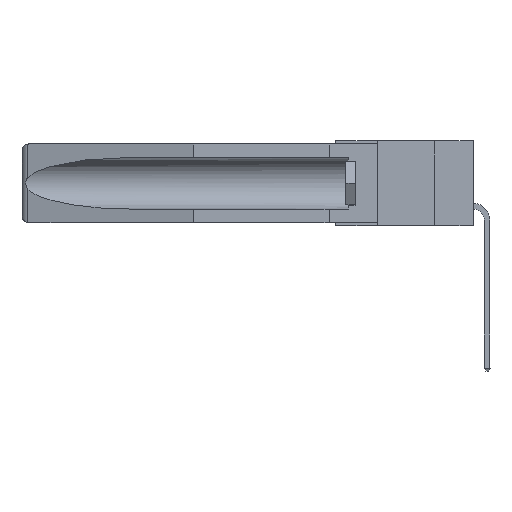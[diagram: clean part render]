
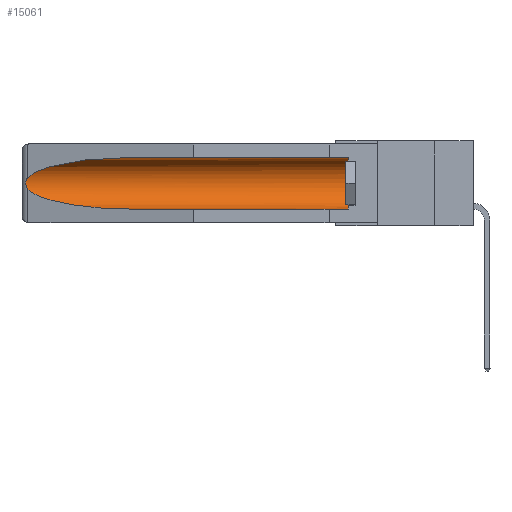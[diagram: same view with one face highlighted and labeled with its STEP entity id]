
A CAD part, left-side view. The second image highlights one B-rep face of the part: STEP entity #15061.
In plain terms, the highlighted cylindrical face has radius 2.857 mm (diameter 5.715 mm), a partial arc.
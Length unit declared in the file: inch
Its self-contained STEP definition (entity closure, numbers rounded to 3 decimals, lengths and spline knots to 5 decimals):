
#56 = VERTEX_POINT ( 'NONE', #14654 ) ;
#414 = AXIS2_PLACEMENT_3D ( 'NONE', #13241, #4403, #14778 ) ;
#901 = CARTESIAN_POINT ( 'NONE',  ( 0.21114, 1.30732, -0.284 ) ) ;
#962 = CARTESIAN_POINT ( 'NONE',  ( 0.25451, 1.48313, -0.09465 ) ) ;
#967 = CARTESIAN_POINT ( 'NONE',  ( 0.155, 1.07973, -0.284 ) ) ;
#1144 = DIRECTION ( 'NONE',  ( 0., 0., 1. ) ) ;
#1234 = FACE_OUTER_BOUND ( 'NONE', #15044, .T. ) ;
#1832 = LINE ( 'NONE', #9757, #6732 ) ;
#2042 = CARTESIAN_POINT ( 'NONE',  ( 0.26537, 1.52718, -0.19328 ) ) ;
#2167 = CARTESIAN_POINT ( 'NONE',  ( 0.26597, 1.52961, -0.15275 ) ) ;
#2314 = CARTESIAN_POINT ( 'NONE',  ( 0.26655, 1.53094, -0.18657 ) ) ;
#3698 = CARTESIAN_POINT ( 'NONE',  ( 0.2673, 1.53269, -0.17917 ) ) ;
#3832 = DIRECTION ( 'NONE',  ( 0., 1., 0. ) ) ;
#3889 = CIRCLE ( 'NONE', #11942, 0.1125 ) ;
#4142 = CARTESIAN_POINT ( 'NONE',  ( 0.26537, 1.52718, -0.14972 ) ) ;
#4305 = VERTEX_POINT ( 'NONE', #18230 ) ;
#4403 = DIRECTION ( 'NONE',  ( 0., 1., 0. ) ) ;
#4667 = LINE ( 'NONE', #8243, #4895 ) ;
#4740 = VERTEX_POINT ( 'NONE', #14899 ) ;
#4895 = VECTOR ( 'NONE', #8170, 39.37008 ) ;
#5308 = CARTESIAN_POINT ( 'NONE',  ( 0.26597, 1.5296, -0.19026 ) ) ;
#6732 = VECTOR ( 'NONE', #3832, 39.37008 ) ;
#6853 =( BOUNDED_CURVE ( )  B_SPLINE_CURVE ( 3, ( #8586, #9779, #901, #967 ),
 .UNSPECIFIED., .F., .T. ) 
 B_SPLINE_CURVE_WITH_KNOTS ( ( 4, 4 ),
 ( 0.1948, 1.5708 ),
 .UNSPECIFIED. ) 
 CURVE ( )  GEOMETRIC_REPRESENTATION_ITEM ( )  RATIONAL_B_SPLINE_CURVE ( ( 1., 0.848, 0.848, 1. ) ) 
 REPRESENTATION_ITEM ( '' )  );
#7014 = ORIENTED_EDGE ( 'NONE', *, *, #17585, .F. ) ;
#8170 = DIRECTION ( 'NONE',  ( 0., 1., 0. ) ) ;
#8243 = CARTESIAN_POINT ( 'NONE',  ( 0.155, -0.30754, -0.059 ) ) ;
#8586 = CARTESIAN_POINT ( 'NONE',  ( 0.26537, 1.52718, -0.19328 ) ) ;
#8675 = ORIENTED_EDGE ( 'NONE', *, *, #17444, .T. ) ;
#9653 = CARTESIAN_POINT ( 'NONE',  ( 0.2675, 1.53308, -0.17534 ) ) ;
#9757 = CARTESIAN_POINT ( 'NONE',  ( 0.155, -0.30754, -0.284 ) ) ;
#9779 = CARTESIAN_POINT ( 'NONE',  ( 0.25451, 1.48313, -0.24835 ) ) ;
#10020 = CARTESIAN_POINT ( 'NONE',  ( 0.155, 0.126, -0.1715 ) ) ;
#10242 =( BOUNDED_CURVE ( )  B_SPLINE_CURVE ( 3, ( #18774, #12919, #962, #4142 ),
 .UNSPECIFIED., .F., .F. ) 
 B_SPLINE_CURVE_WITH_KNOTS ( ( 4, 4 ),
 ( 4.71239, 6.08839 ),
 .UNSPECIFIED. ) 
 CURVE ( )  GEOMETRIC_REPRESENTATION_ITEM ( )  RATIONAL_B_SPLINE_CURVE ( ( 1., 0.848, 0.848, 1. ) ) 
 REPRESENTATION_ITEM ( '' )  );
#10816 = ORIENTED_EDGE ( 'NONE', *, *, #13235, .T. ) ;
#11368 = EDGE_CURVE ( 'NONE', #15249, #56, #14258, .T. ) ;
#11382 = CARTESIAN_POINT ( 'NONE',  ( 0.26537, 1.52718, -0.14972 ) ) ;
#11671 = CYLINDRICAL_SURFACE ( 'NONE', #414, 0.1125 ) ;
#11942 = AXIS2_PLACEMENT_3D ( 'NONE', #10020, #14401, #1144 ) ;
#12246 = ORIENTED_EDGE ( 'NONE', *, *, #17041, .T. ) ;
#12292 = VERTEX_POINT ( 'NONE', #17568 ) ;
#12471 = ORIENTED_EDGE ( 'NONE', *, *, #11368, .T. ) ;
#12919 = CARTESIAN_POINT ( 'NONE',  ( 0.21114, 1.30732, -0.059 ) ) ;
#13235 = EDGE_CURVE ( 'NONE', #4305, #4740, #3889, .T. ) ;
#13241 = CARTESIAN_POINT ( 'NONE',  ( 0.155, -0.30754, -0.1715 ) ) ;
#14030 = CARTESIAN_POINT ( 'NONE',  ( 0.2673, 1.5327, -0.16383 ) ) ;
#14258 = B_SPLINE_CURVE_WITH_KNOTS ( 'NONE', 3,
 ( #15561, #2167, #18468, #14030, #16920, #9653, #3698, #2314, #5308, #2042 ),
 .UNSPECIFIED., .F., .F.,
 ( 4, 2, 2, 2, 4 ),
 ( 0., 0.00029, 0.00058, 0.00087, 0.00117 ),
 .UNSPECIFIED. ) ;
#14401 = DIRECTION ( 'NONE',  ( 0., -1., 0. ) ) ;
#14558 = EDGE_CURVE ( 'NONE', #15714, #15249, #10242, .T. ) ;
#14654 = CARTESIAN_POINT ( 'NONE',  ( 0.26537, 1.52718, -0.19328 ) ) ;
#14778 = DIRECTION ( 'NONE',  ( 0., 0., 1. ) ) ;
#14899 = CARTESIAN_POINT ( 'NONE',  ( 0.155, 0.126, -0.059 ) ) ;
#15044 = EDGE_LOOP ( 'NONE', ( #18968, #12471, #12246, #7014, #10816, #8675 ) ) ;
#15061 = ADVANCED_FACE ( 'NONE', ( #1234 ), #11671, .F. ) ;
#15249 = VERTEX_POINT ( 'NONE', #11382 ) ;
#15561 = CARTESIAN_POINT ( 'NONE',  ( 0.26537, 1.52718, -0.14972 ) ) ;
#15714 = VERTEX_POINT ( 'NONE', #17135 ) ;
#16920 = CARTESIAN_POINT ( 'NONE',  ( 0.2675, 1.53308, -0.16763 ) ) ;
#17041 = EDGE_CURVE ( 'NONE', #56, #12292, #6853, .T. ) ;
#17135 = CARTESIAN_POINT ( 'NONE',  ( 0.155, 1.07973, -0.059 ) ) ;
#17444 = EDGE_CURVE ( 'NONE', #4740, #15714, #4667, .T. ) ;
#17568 = CARTESIAN_POINT ( 'NONE',  ( 0.155, 1.07973, -0.284 ) ) ;
#17585 = EDGE_CURVE ( 'NONE', #4305, #12292, #1832, .T. ) ;
#18230 = CARTESIAN_POINT ( 'NONE',  ( 0.155, 0.126, -0.284 ) ) ;
#18468 = CARTESIAN_POINT ( 'NONE',  ( 0.26654, 1.53092, -0.15636 ) ) ;
#18774 = CARTESIAN_POINT ( 'NONE',  ( 0.155, 1.07973, -0.059 ) ) ;
#18968 = ORIENTED_EDGE ( 'NONE', *, *, #14558, .T. ) ;
